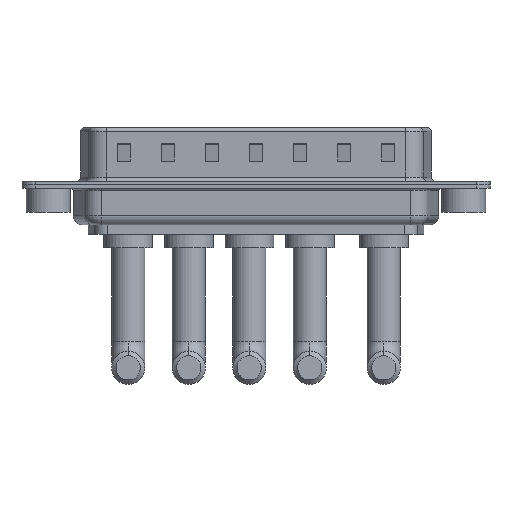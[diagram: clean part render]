
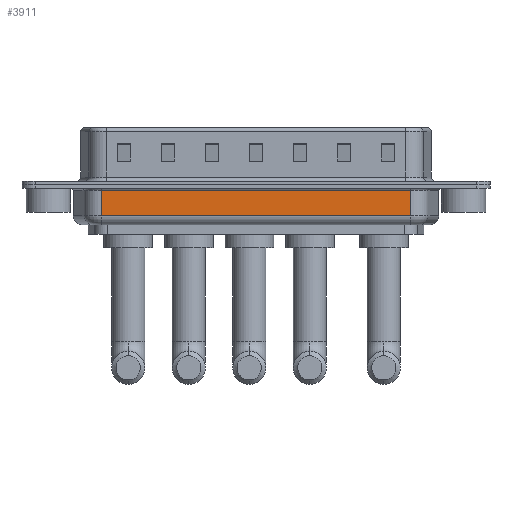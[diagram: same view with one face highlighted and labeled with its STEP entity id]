
A CAD part, front view. The second image highlights one B-rep face of the part: STEP entity #3911.
In plain terms, the highlighted planar face has unit normal (0, -1, 0).
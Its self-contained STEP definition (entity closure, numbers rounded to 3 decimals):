
#261 = CARTESIAN_POINT ( 'NONE',  ( 41.044, -5.35, -3.5 ) ) ;
#446 = CARTESIAN_POINT ( 'NONE',  ( 6.006, -5.35, -3.5 ) ) ;
#515 = CARTESIAN_POINT ( 'NONE',  ( 41.044, -5.35, -4.5 ) ) ;
#658 = LINE ( 'NONE', #515, #8152 ) ;
#3407 = EDGE_CURVE ( 'NONE', #13746, #4702, #9860, .T. ) ;
#3911 = ADVANCED_FACE ( 'NONE', ( #5333 ), #9768, .F. ) ;
#3965 = CARTESIAN_POINT ( 'NONE',  ( 6.006, -5.35, -0.65 ) ) ;
#4178 = CARTESIAN_POINT ( 'NONE',  ( 41.044, -5.35, -0.65 ) ) ;
#4368 = ORIENTED_EDGE ( 'NONE', *, *, #12760, .T. ) ;
#4455 = DIRECTION ( 'NONE',  ( 0., 0., 1. ) ) ;
#4475 = VERTEX_POINT ( 'NONE', #261 ) ;
#4602 = DIRECTION ( 'NONE',  ( 0., 1., 0. ) ) ;
#4702 = VERTEX_POINT ( 'NONE', #3965 ) ;
#4983 = DIRECTION ( 'NONE',  ( 1., 0., 0. ) ) ;
#5333 = FACE_OUTER_BOUND ( 'NONE', #6755, .T. ) ;
#5653 = ORIENTED_EDGE ( 'NONE', *, *, #11604, .T. ) ;
#5732 = VECTOR ( 'NONE', #14167, 1000. ) ;
#6755 = EDGE_LOOP ( 'NONE', ( #11501, #5653, #4368, #14201 ) ) ;
#7132 = LINE ( 'NONE', #7275, #10167 ) ;
#7275 = CARTESIAN_POINT ( 'NONE',  ( 6.006, -5.35, -0.65 ) ) ;
#7394 = LINE ( 'NONE', #446, #12771 ) ;
#7687 = CARTESIAN_POINT ( 'NONE',  ( 6.006, -5.35, -4.5 ) ) ;
#7913 = EDGE_CURVE ( 'NONE', #14162, #4702, #7132, .T. ) ;
#8152 = VECTOR ( 'NONE', #13003, 1000. ) ;
#8691 = CARTESIAN_POINT ( 'NONE',  ( 6.006, -5.35, -4.5 ) ) ;
#9768 = PLANE ( 'NONE',  #13312 ) ;
#9802 = CARTESIAN_POINT ( 'NONE',  ( 6.006, -5.35, -3.5 ) ) ;
#9860 = LINE ( 'NONE', #7687, #5732 ) ;
#10167 = VECTOR ( 'NONE', #11585, 1000. ) ;
#11501 = ORIENTED_EDGE ( 'NONE', *, *, #3407, .F. ) ;
#11585 = DIRECTION ( 'NONE',  ( -1., 0., 0. ) ) ;
#11604 = EDGE_CURVE ( 'NONE', #13746, #4475, #7394, .T. ) ;
#12760 = EDGE_CURVE ( 'NONE', #4475, #14162, #658, .T. ) ;
#12771 = VECTOR ( 'NONE', #4983, 1000. ) ;
#13003 = DIRECTION ( 'NONE',  ( 0., 0., 1. ) ) ;
#13312 = AXIS2_PLACEMENT_3D ( 'NONE', #8691, #4602, #4455 ) ;
#13746 = VERTEX_POINT ( 'NONE', #9802 ) ;
#14162 = VERTEX_POINT ( 'NONE', #4178 ) ;
#14167 = DIRECTION ( 'NONE',  ( 0., 0., 1. ) ) ;
#14201 = ORIENTED_EDGE ( 'NONE', *, *, #7913, .T. ) ;
